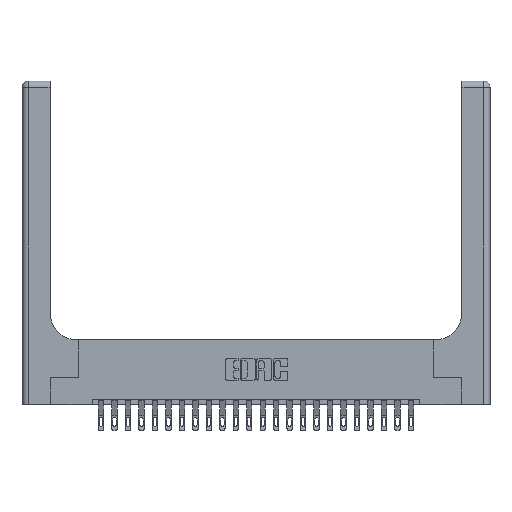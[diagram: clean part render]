
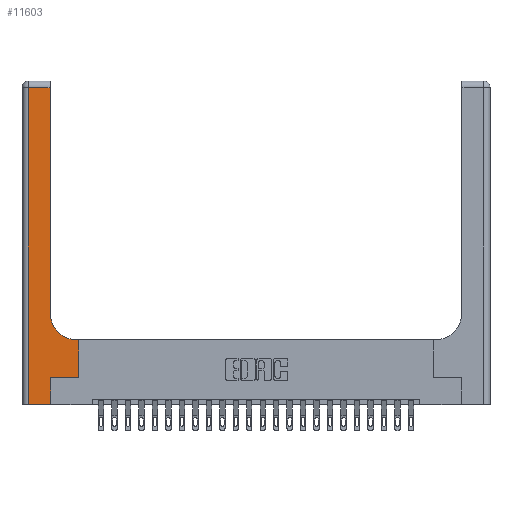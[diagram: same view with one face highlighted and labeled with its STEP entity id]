
A CAD part, top view. The second image highlights one B-rep face of the part: STEP entity #11603.
In plain terms, the highlighted planar face has unit normal (0, 0, 1).
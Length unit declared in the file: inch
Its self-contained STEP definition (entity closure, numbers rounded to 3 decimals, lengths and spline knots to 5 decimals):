
#1446 = VECTOR ( 'NONE', #14244, 39.37008 ) ;
#1617 = CARTESIAN_POINT ( 'NONE',  ( 0.26, 0.85, 0.37 ) ) ;
#1668 = DIRECTION ( 'NONE',  ( 0., 0., -1. ) ) ;
#2020 = DIRECTION ( 'NONE',  ( 1., 0., 0. ) ) ;
#2109 = ORIENTED_EDGE ( 'NONE', *, *, #3924, .T. ) ;
#2166 = VERTEX_POINT ( 'NONE', #1617 ) ;
#2370 = EDGE_CURVE ( 'NONE', #18515, #19426, #12290, .T. ) ;
#2435 = CARTESIAN_POINT ( 'NONE',  ( 0.265, 0., 0.37 ) ) ;
#2487 = FACE_OUTER_BOUND ( 'NONE', #21268, .T. ) ;
#3508 = CARTESIAN_POINT ( 'NONE',  ( 0.51, 0.85, 0.37 ) ) ;
#3924 = EDGE_CURVE ( 'NONE', #19426, #18644, #18843, .T. ) ;
#3988 = CARTESIAN_POINT ( 'NONE',  ( 0., 0., 0.37 ) ) ;
#4377 = LINE ( 'NONE', #21271, #20151 ) ;
#4687 = CARTESIAN_POINT ( 'NONE',  ( 0.06, 2.94, 0.37 ) ) ;
#5577 = ORIENTED_EDGE ( 'NONE', *, *, #22676, .T. ) ;
#6455 = CARTESIAN_POINT ( 'NONE',  ( 0.528, 0.25, 0.37 ) ) ;
#6900 = LINE ( 'NONE', #23695, #10483 ) ;
#7399 = LINE ( 'NONE', #3988, #16315 ) ;
#8089 = CARTESIAN_POINT ( 'NONE',  ( 0.528, 0.6, 0.37 ) ) ;
#8264 = DIRECTION ( 'NONE',  ( -1., 0., 0. ) ) ;
#8992 = VECTOR ( 'NONE', #19601, 39.37008 ) ;
#9277 = VECTOR ( 'NONE', #13631, 39.37008 ) ;
#9382 = CARTESIAN_POINT ( 'NONE',  ( 0.528, 0.25, 0.37 ) ) ;
#9492 = VERTEX_POINT ( 'NONE', #2435 ) ;
#9856 = CARTESIAN_POINT ( 'NONE',  ( 0.26, 0.6, 0.37 ) ) ;
#10371 = VERTEX_POINT ( 'NONE', #4687 ) ;
#10483 = VECTOR ( 'NONE', #14820, 39.37008 ) ;
#10709 = VERTEX_POINT ( 'NONE', #20482 ) ;
#11227 = AXIS2_PLACEMENT_3D ( 'NONE', #11757, #17824, #12228 ) ;
#11603 = ADVANCED_FACE ( 'NONE', ( #2487 ), #19410, .F. ) ;
#11714 = ORIENTED_EDGE ( 'NONE', *, *, #17662, .T. ) ;
#11757 = CARTESIAN_POINT ( 'NONE',  ( 0., 3., 0.37 ) ) ;
#11995 = CIRCLE ( 'NONE', #22855, 0.25 ) ;
#12228 = DIRECTION ( 'NONE',  ( -1., 0., 0. ) ) ;
#12290 = LINE ( 'NONE', #17398, #8992 ) ;
#13063 = VECTOR ( 'NONE', #16406, 39.37008 ) ;
#13631 = DIRECTION ( 'NONE',  ( -1., 0., 0. ) ) ;
#14244 = DIRECTION ( 'NONE',  ( 0., 1., 0. ) ) ;
#14421 = ORIENTED_EDGE ( 'NONE', *, *, #2370, .T. ) ;
#14540 = ORIENTED_EDGE ( 'NONE', *, *, #21429, .T. ) ;
#14820 = DIRECTION ( 'NONE',  ( 0., 1., 0. ) ) ;
#14942 = DIRECTION ( 'NONE',  ( 1., 0., 0. ) ) ;
#15434 = LINE ( 'NONE', #9856, #9277 ) ;
#15926 = CARTESIAN_POINT ( 'NONE',  ( 0.06, 3., 0.37 ) ) ;
#15946 = VERTEX_POINT ( 'NONE', #18996 ) ;
#16315 = VECTOR ( 'NONE', #14942, 39.37008 ) ;
#16406 = DIRECTION ( 'NONE',  ( 0., -1., 0. ) ) ;
#16656 = EDGE_CURVE ( 'NONE', #2166, #15946, #17517, .T. ) ;
#16728 = ORIENTED_EDGE ( 'NONE', *, *, #19886, .T. ) ;
#16861 = ORIENTED_EDGE ( 'NONE', *, *, #16656, .T. ) ;
#17398 = CARTESIAN_POINT ( 'NONE',  ( 0.265, 0.25, 0.37 ) ) ;
#17517 = LINE ( 'NONE', #17895, #1446 ) ;
#17662 = EDGE_CURVE ( 'NONE', #15946, #10371, #4377, .T. ) ;
#17749 = EDGE_CURVE ( 'NONE', #18644, #20025, #15434, .T. ) ;
#17824 = DIRECTION ( 'NONE',  ( 0., 0., -1. ) ) ;
#17895 = CARTESIAN_POINT ( 'NONE',  ( 0.26, 3., 0.37 ) ) ;
#18430 = EDGE_CURVE ( 'NONE', #9492, #18515, #6900, .T. ) ;
#18515 = VERTEX_POINT ( 'NONE', #19035 ) ;
#18644 = VERTEX_POINT ( 'NONE', #8089 ) ;
#18843 = LINE ( 'NONE', #9382, #19808 ) ;
#18996 = CARTESIAN_POINT ( 'NONE',  ( 0.26, 2.94, 0.37 ) ) ;
#19035 = CARTESIAN_POINT ( 'NONE',  ( 0.265, 0.25, 0.37 ) ) ;
#19410 = PLANE ( 'NONE',  #11227 ) ;
#19426 = VERTEX_POINT ( 'NONE', #6455 ) ;
#19601 = DIRECTION ( 'NONE',  ( 1., 0., 0. ) ) ;
#19683 = LINE ( 'NONE', #15926, #13063 ) ;
#19808 = VECTOR ( 'NONE', #20695, 39.37008 ) ;
#19886 = EDGE_CURVE ( 'NONE', #10709, #9492, #7399, .T. ) ;
#20025 = VERTEX_POINT ( 'NONE', #23902 ) ;
#20151 = VECTOR ( 'NONE', #8264, 39.37008 ) ;
#20339 = ORIENTED_EDGE ( 'NONE', *, *, #17749, .T. ) ;
#20390 = ORIENTED_EDGE ( 'NONE', *, *, #18430, .T. ) ;
#20482 = CARTESIAN_POINT ( 'NONE',  ( 0.06, 0., 0.37 ) ) ;
#20695 = DIRECTION ( 'NONE',  ( 0., 1., 0. ) ) ;
#21268 = EDGE_LOOP ( 'NONE', ( #16861, #11714, #14540, #16728, #20390, #14421, #2109, #20339, #5577 ) ) ;
#21271 = CARTESIAN_POINT ( 'NONE',  ( 0., 2.94, 0.37 ) ) ;
#21429 = EDGE_CURVE ( 'NONE', #10371, #10709, #19683, .T. ) ;
#22676 = EDGE_CURVE ( 'NONE', #20025, #2166, #11995, .T. ) ;
#22855 = AXIS2_PLACEMENT_3D ( 'NONE', #3508, #1668, #2020 ) ;
#23695 = CARTESIAN_POINT ( 'NONE',  ( 0.265, 0., 0.37 ) ) ;
#23902 = CARTESIAN_POINT ( 'NONE',  ( 0.51, 0.6, 0.37 ) ) ;
